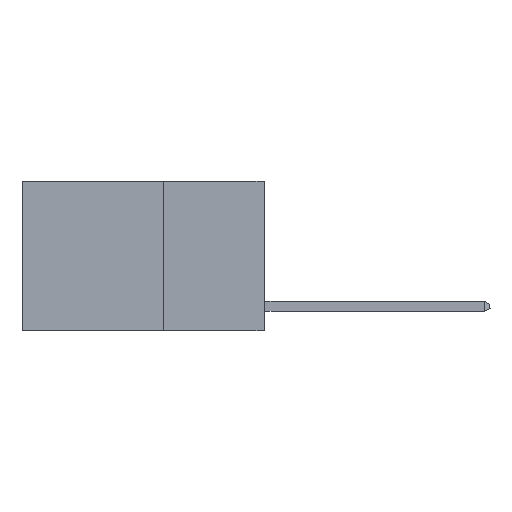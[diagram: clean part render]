
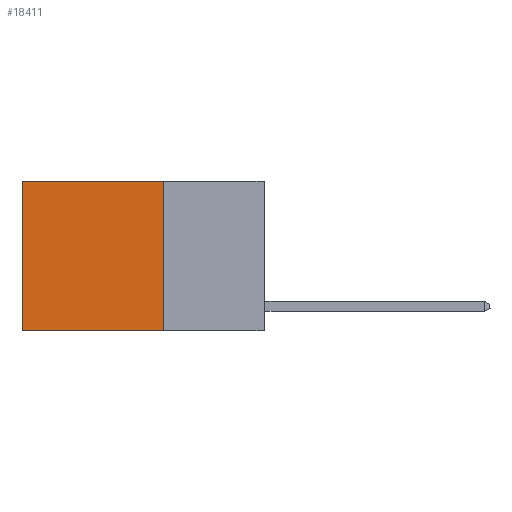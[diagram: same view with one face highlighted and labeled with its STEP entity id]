
A CAD part, left-side view. The second image highlights one B-rep face of the part: STEP entity #18411.
In plain terms, the highlighted planar face has unit normal (-1, 0, 0).
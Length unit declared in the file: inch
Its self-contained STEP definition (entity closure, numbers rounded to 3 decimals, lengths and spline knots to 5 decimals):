
#208 = DIRECTION ( 'NONE',  ( 0., 0., -1. ) ) ;
#669 = ORIENTED_EDGE ( 'NONE', *, *, #14219, .T. ) ;
#1061 = CARTESIAN_POINT ( 'NONE',  ( 0.2625, 0.25, -0.37 ) ) ;
#1614 = EDGE_CURVE ( 'NONE', #17440, #20613, #8760, .T. ) ;
#1815 = CARTESIAN_POINT ( 'NONE',  ( 0.2625, 0.6, 0. ) ) ;
#2598 = CARTESIAN_POINT ( 'NONE',  ( 0.2625, 0.6, -0.37 ) ) ;
#5986 = EDGE_CURVE ( 'NONE', #6447, #20613, #16200, .T. ) ;
#6007 = DIRECTION ( 'NONE',  ( 0., 0., -1. ) ) ;
#6027 = VERTEX_POINT ( 'NONE', #9342 ) ;
#6447 = VERTEX_POINT ( 'NONE', #14695 ) ;
#7825 = LINE ( 'NONE', #9293, #14831 ) ;
#8760 = LINE ( 'NONE', #1815, #13279 ) ;
#8859 = DIRECTION ( 'NONE',  ( 0., 0., -1. ) ) ;
#8931 = CARTESIAN_POINT ( 'NONE',  ( 0.2625, 0.25, 0. ) ) ;
#9293 = CARTESIAN_POINT ( 'NONE',  ( 0.2625, 0.25, 0. ) ) ;
#9342 = CARTESIAN_POINT ( 'NONE',  ( 0.2625, 0.25, 0. ) ) ;
#10560 = CARTESIAN_POINT ( 'NONE',  ( 0.2625, 0.6, 0. ) ) ;
#10841 = PLANE ( 'NONE',  #13208 ) ;
#11984 = LINE ( 'NONE', #12413, #19320 ) ;
#12413 = CARTESIAN_POINT ( 'NONE',  ( 0.2625, 0.25, 0. ) ) ;
#12675 = DIRECTION ( 'NONE',  ( 0., 1., 0. ) ) ;
#13208 = AXIS2_PLACEMENT_3D ( 'NONE', #8931, #15780, #6007 ) ;
#13279 = VECTOR ( 'NONE', #8859, 39.37008 ) ;
#13596 = VECTOR ( 'NONE', #16408, 39.37008 ) ;
#14219 = EDGE_CURVE ( 'NONE', #6027, #17440, #7825, .T. ) ;
#14538 = FACE_OUTER_BOUND ( 'NONE', #21398, .T. ) ;
#14695 = CARTESIAN_POINT ( 'NONE',  ( 0.2625, 0.25, -0.37 ) ) ;
#14831 = VECTOR ( 'NONE', #12675, 39.37008 ) ;
#15780 = DIRECTION ( 'NONE',  ( 1., 0., 0. ) ) ;
#16200 = LINE ( 'NONE', #1061, #13596 ) ;
#16401 = ORIENTED_EDGE ( 'NONE', *, *, #5986, .F. ) ;
#16408 = DIRECTION ( 'NONE',  ( 0., 1., 0. ) ) ;
#17440 = VERTEX_POINT ( 'NONE', #10560 ) ;
#18411 = ADVANCED_FACE ( 'NONE', ( #14538 ), #10841, .F. ) ;
#19320 = VECTOR ( 'NONE', #208, 39.37008 ) ;
#19552 = EDGE_CURVE ( 'NONE', #6027, #6447, #11984, .T. ) ;
#19840 = ORIENTED_EDGE ( 'NONE', *, *, #19552, .F. ) ;
#20613 = VERTEX_POINT ( 'NONE', #2598 ) ;
#20734 = ORIENTED_EDGE ( 'NONE', *, *, #1614, .T. ) ;
#21398 = EDGE_LOOP ( 'NONE', ( #20734, #16401, #19840, #669 ) ) ;
